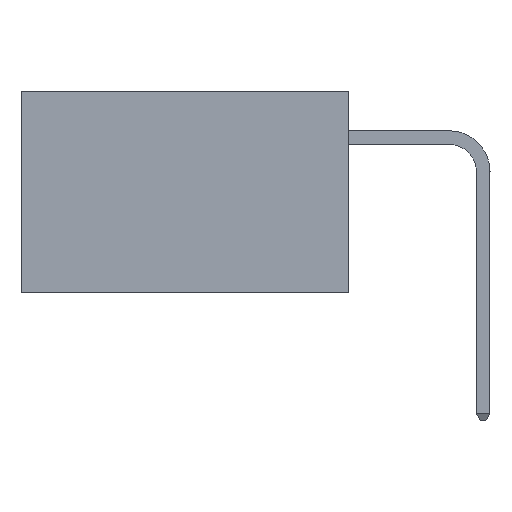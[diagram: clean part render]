
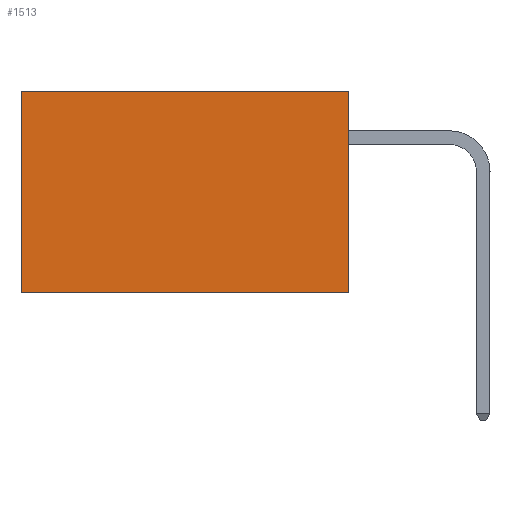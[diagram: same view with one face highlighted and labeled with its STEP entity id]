
A CAD part, left-side view. The second image highlights one B-rep face of the part: STEP entity #1513.
In plain terms, the highlighted planar face has unit normal (-1, 0, 0).
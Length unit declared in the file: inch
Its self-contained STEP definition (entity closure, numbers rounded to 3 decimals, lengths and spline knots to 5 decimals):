
#1513 = ADVANCED_FACE ( 'NONE', ( #18355 ), #31241, .F. ) ;
#2412 = LINE ( 'NONE', #12656, #17987 ) ;
#2805 = CARTESIAN_POINT ( 'NONE',  ( 0.2875, 0., -0.37 ) ) ;
#2955 = VERTEX_POINT ( 'NONE', #15404 ) ;
#4060 = EDGE_LOOP ( 'NONE', ( #15574, #10744, #29940, #35406 ) ) ;
#4288 = EDGE_CURVE ( 'NONE', #38824, #2955, #5042, .T. ) ;
#4974 = LINE ( 'NONE', #15545, #37401 ) ;
#5042 = LINE ( 'NONE', #13706, #28483 ) ;
#7033 = LINE ( 'NONE', #21912, #37491 ) ;
#8873 = EDGE_CURVE ( 'NONE', #16128, #28978, #4974, .T. ) ;
#9810 = CARTESIAN_POINT ( 'NONE',  ( 0.2875, 0., 0. ) ) ;
#10744 = ORIENTED_EDGE ( 'NONE', *, *, #23070, .F. ) ;
#12656 = CARTESIAN_POINT ( 'NONE',  ( 0.2875, 0., -0.37 ) ) ;
#13706 = CARTESIAN_POINT ( 'NONE',  ( 0.2875, 0.6, 0. ) ) ;
#15202 = DIRECTION ( 'NONE',  ( 1., 0., 0. ) ) ;
#15404 = CARTESIAN_POINT ( 'NONE',  ( 0.2875, 0.6, -0.37 ) ) ;
#15545 = CARTESIAN_POINT ( 'NONE',  ( 0.2875, 0., 0. ) ) ;
#15574 = ORIENTED_EDGE ( 'NONE', *, *, #4288, .T. ) ;
#15786 = DIRECTION ( 'NONE',  ( 0., 1., 0. ) ) ;
#16128 = VERTEX_POINT ( 'NONE', #9810 ) ;
#17472 = CARTESIAN_POINT ( 'NONE',  ( 0.2875, 0., 0. ) ) ;
#17987 = VECTOR ( 'NONE', #15786, 39.37008 ) ;
#18355 = FACE_OUTER_BOUND ( 'NONE', #4060, .T. ) ;
#19874 = DIRECTION ( 'NONE',  ( 0., 0., -1. ) ) ;
#21912 = CARTESIAN_POINT ( 'NONE',  ( 0.2875, 0., 0. ) ) ;
#23070 = EDGE_CURVE ( 'NONE', #28978, #2955, #2412, .T. ) ;
#24611 = AXIS2_PLACEMENT_3D ( 'NONE', #17472, #15202, #33548 ) ;
#27438 = CARTESIAN_POINT ( 'NONE',  ( 0.2875, 0.6, 0. ) ) ;
#27808 = DIRECTION ( 'NONE',  ( 0., 1., 0. ) ) ;
#28483 = VECTOR ( 'NONE', #19874, 39.37008 ) ;
#28978 = VERTEX_POINT ( 'NONE', #2805 ) ;
#29940 = ORIENTED_EDGE ( 'NONE', *, *, #8873, .F. ) ;
#31241 = PLANE ( 'NONE',  #24611 ) ;
#33548 = DIRECTION ( 'NONE',  ( 0., 0., -1. ) ) ;
#35406 = ORIENTED_EDGE ( 'NONE', *, *, #36901, .T. ) ;
#36679 = DIRECTION ( 'NONE',  ( 0., 0., -1. ) ) ;
#36901 = EDGE_CURVE ( 'NONE', #16128, #38824, #7033, .T. ) ;
#37401 = VECTOR ( 'NONE', #36679, 39.37008 ) ;
#37491 = VECTOR ( 'NONE', #27808, 39.37008 ) ;
#38824 = VERTEX_POINT ( 'NONE', #27438 ) ;
